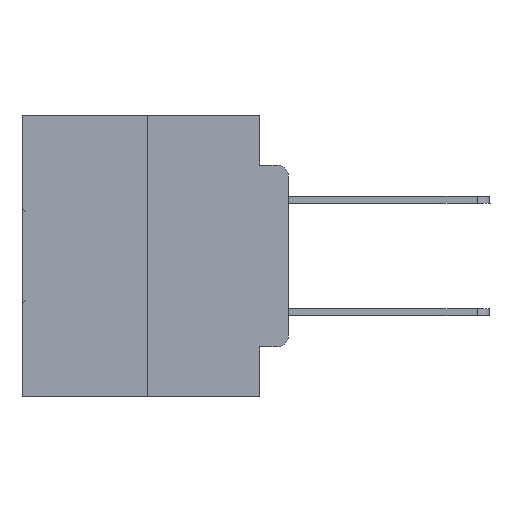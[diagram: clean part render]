
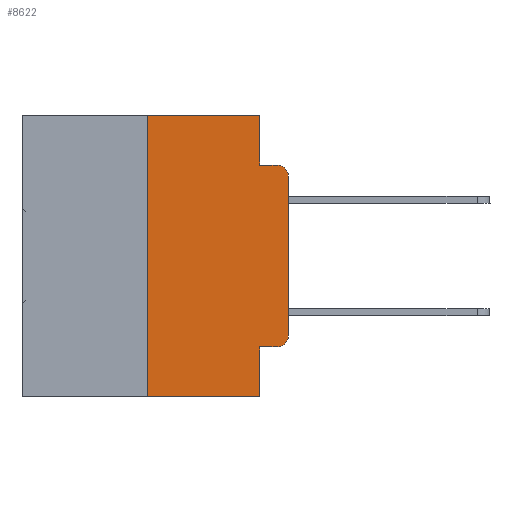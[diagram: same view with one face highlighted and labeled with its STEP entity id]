
A CAD part, left-side view. The second image highlights one B-rep face of the part: STEP entity #8622.
In plain terms, the highlighted planar face has unit normal (-1, 0, 0).
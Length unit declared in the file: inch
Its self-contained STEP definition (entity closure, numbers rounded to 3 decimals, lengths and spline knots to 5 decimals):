
#173 = CARTESIAN_POINT ( 'NONE',  ( 0., 0.473, 0. ) ) ;
#184 = EDGE_CURVE ( 'NONE', #5630, #19977, #16390, .T. ) ;
#205 = VECTOR ( 'NONE', #17262, 39.37008 ) ;
#414 = ORIENTED_EDGE ( 'NONE', *, *, #24261, .F. ) ;
#2904 = VERTEX_POINT ( 'NONE', #20201 ) ;
#3300 = VERTEX_POINT ( 'NONE', #28028 ) ;
#3585 = CARTESIAN_POINT ( 'NONE',  ( 0., 0.051, -0.0885 ) ) ;
#3909 = EDGE_LOOP ( 'NONE', ( #10871, #22837, #26381, #414, #18316, #24362, #22296, #29397, #25588, #5153 ) ) ;
#4633 = EDGE_CURVE ( 'NONE', #31624, #20029, #12115, .T. ) ;
#4655 = CIRCLE ( 'NONE', #17548, 0.02 ) ;
#5153 = ORIENTED_EDGE ( 'NONE', *, *, #19608, .T. ) ;
#5630 = VERTEX_POINT ( 'NONE', #17611 ) ;
#6427 = CARTESIAN_POINT ( 'NONE',  ( 0., 0.25, 0. ) ) ;
#7104 = EDGE_CURVE ( 'NONE', #26836, #20029, #20483, .T. ) ;
#7742 = EDGE_CURVE ( 'NONE', #31624, #3300, #29064, .T. ) ;
#7833 = CARTESIAN_POINT ( 'NONE',  ( 0., 0.051, -0.5 ) ) ;
#8026 = DIRECTION ( 'NONE',  ( 0., 0., -1. ) ) ;
#8551 = FACE_OUTER_BOUND ( 'NONE', #3909, .T. ) ;
#8622 = ADVANCED_FACE ( 'NONE', ( #8551 ), #31931, .F. ) ;
#9170 = LINE ( 'NONE', #3585, #205 ) ;
#9462 = VECTOR ( 'NONE', #26046, 39.37008 ) ;
#9609 = CARTESIAN_POINT ( 'NONE',  ( 0., 0., -0.1085 ) ) ;
#9876 = CARTESIAN_POINT ( 'NONE',  ( 0., 0.02, -0.1085 ) ) ;
#10856 = DIRECTION ( 'NONE',  ( 0., -1., 0. ) ) ;
#10871 = ORIENTED_EDGE ( 'NONE', *, *, #184, .T. ) ;
#12115 = LINE ( 'NONE', #20506, #32075 ) ;
#12249 = CIRCLE ( 'NONE', #26251, 0.02 ) ;
#12262 = DIRECTION ( 'NONE',  ( 0., -1., 0. ) ) ;
#13317 = CARTESIAN_POINT ( 'NONE',  ( 0., 0.051, 0. ) ) ;
#13432 = DIRECTION ( 'NONE',  ( 0., -1., 0. ) ) ;
#13749 = CARTESIAN_POINT ( 'NONE',  ( 0., 0., 0. ) ) ;
#13824 = CARTESIAN_POINT ( 'NONE',  ( 0., 0.473, 0. ) ) ;
#15462 = VECTOR ( 'NONE', #30085, 39.37008 ) ;
#15615 = DIRECTION ( 'NONE',  ( -1., 0., 0. ) ) ;
#16390 = LINE ( 'NONE', #13749, #15462 ) ;
#17104 = CARTESIAN_POINT ( 'NONE',  ( 0., 0.051, -0.0885 ) ) ;
#17173 = AXIS2_PLACEMENT_3D ( 'NONE', #13824, #21519, #8026 ) ;
#17262 = DIRECTION ( 'NONE',  ( 0., -1., 0. ) ) ;
#17532 = CARTESIAN_POINT ( 'NONE',  ( 0., 0.051, -0.4115 ) ) ;
#17548 = AXIS2_PLACEMENT_3D ( 'NONE', #9876, #25678, #17969 ) ;
#17611 = CARTESIAN_POINT ( 'NONE',  ( 0., 0., -0.3915 ) ) ;
#17969 = DIRECTION ( 'NONE',  ( 0., 0., -1. ) ) ;
#18316 = ORIENTED_EDGE ( 'NONE', *, *, #19633, .F. ) ;
#18636 = EDGE_CURVE ( 'NONE', #26836, #33426, #28686, .T. ) ;
#18741 = LINE ( 'NONE', #13317, #19196 ) ;
#19196 = VECTOR ( 'NONE', #23999, 39.37008 ) ;
#19608 = EDGE_CURVE ( 'NONE', #3300, #5630, #12249, .T. ) ;
#19633 = EDGE_CURVE ( 'NONE', #33426, #29980, #24358, .T. ) ;
#19977 = VERTEX_POINT ( 'NONE', #9609 ) ;
#20029 = VERTEX_POINT ( 'NONE', #7833 ) ;
#20201 = CARTESIAN_POINT ( 'NONE',  ( 0., 0.02, -0.0885 ) ) ;
#20483 = LINE ( 'NONE', #29107, #20976 ) ;
#20506 = CARTESIAN_POINT ( 'NONE',  ( 0., 0.051, 0. ) ) ;
#20976 = VECTOR ( 'NONE', #12262, 39.37008 ) ;
#21519 = DIRECTION ( 'NONE',  ( 1., 0., 0. ) ) ;
#21537 = CARTESIAN_POINT ( 'NONE',  ( 0., 0.02, -0.3915 ) ) ;
#22296 = ORIENTED_EDGE ( 'NONE', *, *, #7104, .T. ) ;
#22837 = ORIENTED_EDGE ( 'NONE', *, *, #30904, .T. ) ;
#23291 = CARTESIAN_POINT ( 'NONE',  ( 0., 0.051, 0. ) ) ;
#23428 = VECTOR ( 'NONE', #10856, 39.37008 ) ;
#23999 = DIRECTION ( 'NONE',  ( 0., 0., -1. ) ) ;
#24261 = EDGE_CURVE ( 'NONE', #29980, #27696, #18741, .T. ) ;
#24358 = LINE ( 'NONE', #173, #23428 ) ;
#24362 = ORIENTED_EDGE ( 'NONE', *, *, #18636, .F. ) ;
#25588 = ORIENTED_EDGE ( 'NONE', *, *, #7742, .T. ) ;
#25678 = DIRECTION ( 'NONE',  ( -1., 0., 0. ) ) ;
#26046 = DIRECTION ( 'NONE',  ( 0., 0., 1. ) ) ;
#26251 = AXIS2_PLACEMENT_3D ( 'NONE', #21537, #15615, #34603 ) ;
#26381 = ORIENTED_EDGE ( 'NONE', *, *, #26567, .F. ) ;
#26567 = EDGE_CURVE ( 'NONE', #27696, #2904, #9170, .T. ) ;
#26647 = VECTOR ( 'NONE', #13432, 39.37008 ) ;
#26836 = VERTEX_POINT ( 'NONE', #33728 ) ;
#27696 = VERTEX_POINT ( 'NONE', #17104 ) ;
#28028 = CARTESIAN_POINT ( 'NONE',  ( 0., 0.02, -0.4115 ) ) ;
#28075 = DIRECTION ( 'NONE',  ( 0., 0., -1. ) ) ;
#28686 = LINE ( 'NONE', #28865, #9462 ) ;
#28865 = CARTESIAN_POINT ( 'NONE',  ( 0., 0.25, 0. ) ) ;
#29064 = LINE ( 'NONE', #31713, #26647 ) ;
#29107 = CARTESIAN_POINT ( 'NONE',  ( 0., 0.473, -0.5 ) ) ;
#29397 = ORIENTED_EDGE ( 'NONE', *, *, #4633, .F. ) ;
#29980 = VERTEX_POINT ( 'NONE', #23291 ) ;
#30085 = DIRECTION ( 'NONE',  ( 0., 0., 1. ) ) ;
#30904 = EDGE_CURVE ( 'NONE', #19977, #2904, #4655, .T. ) ;
#31624 = VERTEX_POINT ( 'NONE', #17532 ) ;
#31713 = CARTESIAN_POINT ( 'NONE',  ( 0., 0.051, -0.4115 ) ) ;
#31931 = PLANE ( 'NONE',  #17173 ) ;
#32075 = VECTOR ( 'NONE', #28075, 39.37008 ) ;
#33426 = VERTEX_POINT ( 'NONE', #6427 ) ;
#33728 = CARTESIAN_POINT ( 'NONE',  ( 0., 0.25, -0.5 ) ) ;
#34603 = DIRECTION ( 'NONE',  ( 0., 0., -1. ) ) ;
